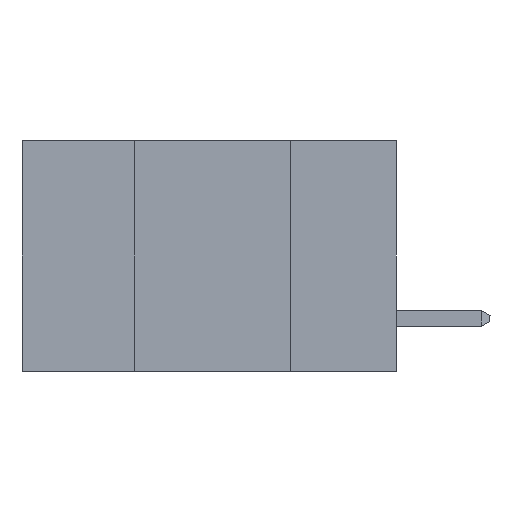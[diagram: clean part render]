
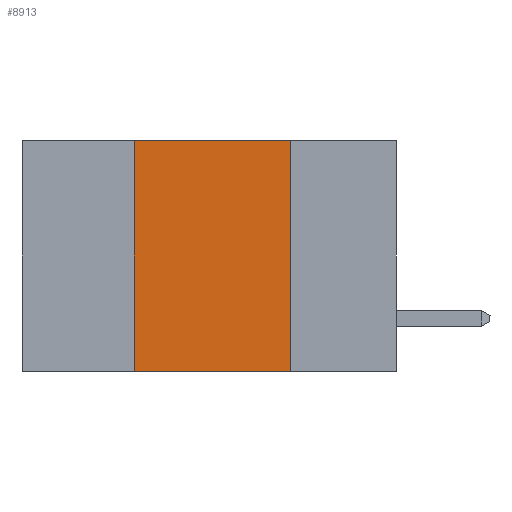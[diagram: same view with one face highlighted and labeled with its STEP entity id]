
A CAD part, left-side view. The second image highlights one B-rep face of the part: STEP entity #8913.
In plain terms, the highlighted planar face has unit normal (-1, 0, 0).
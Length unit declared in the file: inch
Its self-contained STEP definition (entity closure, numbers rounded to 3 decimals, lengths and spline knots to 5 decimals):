
#112 = VERTEX_POINT ( 'NONE', #6037 ) ;
#391 = CARTESIAN_POINT ( 'NONE',  ( 0., 0.17, 0. ) ) ;
#545 = LINE ( 'NONE', #11041, #3199 ) ;
#814 = VECTOR ( 'NONE', #5826, 39.37008 ) ;
#1111 = CARTESIAN_POINT ( 'NONE',  ( 0., 0.17, -0.37 ) ) ;
#1142 = LINE ( 'NONE', #8501, #814 ) ;
#2756 = CARTESIAN_POINT ( 'NONE',  ( 0., 0.6, 0. ) ) ;
#3003 = CARTESIAN_POINT ( 'NONE',  ( 0., 0.6, 0. ) ) ;
#3199 = VECTOR ( 'NONE', #4669, 39.37008 ) ;
#3563 = FACE_OUTER_BOUND ( 'NONE', #11797, .T. ) ;
#3718 = DIRECTION ( 'NONE',  ( 1., 0., 0. ) ) ;
#4397 = AXIS2_PLACEMENT_3D ( 'NONE', #2756, #3718, #10109 ) ;
#4669 = DIRECTION ( 'NONE',  ( 0., -1., 0. ) ) ;
#4720 = VERTEX_POINT ( 'NONE', #9341 ) ;
#5331 = EDGE_CURVE ( 'NONE', #4720, #11672, #545, .T. ) ;
#5778 = VERTEX_POINT ( 'NONE', #391 ) ;
#5826 = DIRECTION ( 'NONE',  ( 0., 0., -1. ) ) ;
#5967 = EDGE_CURVE ( 'NONE', #4720, #112, #8671, .T. ) ;
#6037 = CARTESIAN_POINT ( 'NONE',  ( 0., 0.42, 0. ) ) ;
#6301 = VECTOR ( 'NONE', #12032, 39.37008 ) ;
#6611 = EDGE_CURVE ( 'NONE', #112, #5778, #10920, .T. ) ;
#7208 = EDGE_CURVE ( 'NONE', #5778, #11672, #1142, .T. ) ;
#7365 = ORIENTED_EDGE ( 'NONE', *, *, #5967, .F. ) ;
#7680 = DIRECTION ( 'NONE',  ( 0., -1., 0. ) ) ;
#8501 = CARTESIAN_POINT ( 'NONE',  ( 0., 0.17, -0.37 ) ) ;
#8671 = LINE ( 'NONE', #9351, #6301 ) ;
#8913 = ADVANCED_FACE ( 'NONE', ( #3563 ), #10067, .F. ) ;
#9341 = CARTESIAN_POINT ( 'NONE',  ( 0., 0.42, -0.37 ) ) ;
#9351 = CARTESIAN_POINT ( 'NONE',  ( 0., 0.42, -0.37 ) ) ;
#9718 = ORIENTED_EDGE ( 'NONE', *, *, #5331, .T. ) ;
#10067 = PLANE ( 'NONE',  #4397 ) ;
#10109 = DIRECTION ( 'NONE',  ( 0., 0., -1. ) ) ;
#10353 = VECTOR ( 'NONE', #7680, 39.37008 ) ;
#10920 = LINE ( 'NONE', #3003, #10353 ) ;
#11041 = CARTESIAN_POINT ( 'NONE',  ( 0., 0.6, -0.37 ) ) ;
#11551 = ORIENTED_EDGE ( 'NONE', *, *, #7208, .F. ) ;
#11672 = VERTEX_POINT ( 'NONE', #1111 ) ;
#11797 = EDGE_LOOP ( 'NONE', ( #11551, #11807, #7365, #9718 ) ) ;
#11807 = ORIENTED_EDGE ( 'NONE', *, *, #6611, .F. ) ;
#12032 = DIRECTION ( 'NONE',  ( 0., 0., 1. ) ) ;
